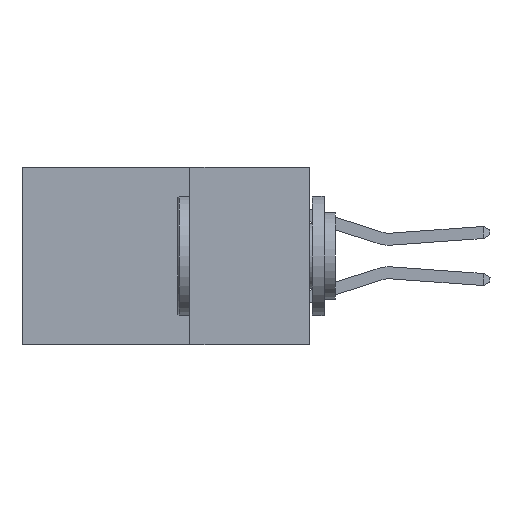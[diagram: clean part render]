
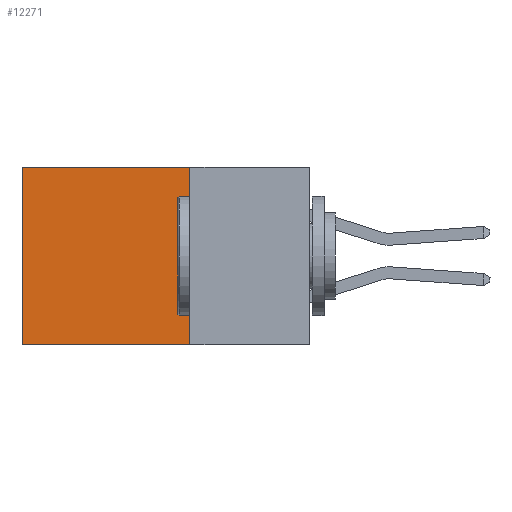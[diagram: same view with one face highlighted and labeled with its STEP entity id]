
A CAD part, left-side view. The second image highlights one B-rep face of the part: STEP entity #12271.
In plain terms, the highlighted planar face has unit normal (-1, 0, 0).
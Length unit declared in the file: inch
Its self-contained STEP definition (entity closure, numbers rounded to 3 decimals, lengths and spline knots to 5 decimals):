
#92 = FACE_OUTER_BOUND ( 'NONE', #14723, .T. ) ;
#436 = CARTESIAN_POINT ( 'NONE',  ( 0.298, 0.25, 0. ) ) ;
#890 = EDGE_CURVE ( 'NONE', #21986, #11920, #2516, .T. ) ;
#1417 = DIRECTION ( 'NONE',  ( 0., 1., 0. ) ) ;
#2134 = DIRECTION ( 'NONE',  ( 0., 0., -1. ) ) ;
#2202 = LINE ( 'NONE', #16030, #6940 ) ;
#2398 = VECTOR ( 'NONE', #1417, 39.37008 ) ;
#2516 = LINE ( 'NONE', #6016, #17220 ) ;
#2739 = CARTESIAN_POINT ( 'NONE',  ( 0.298, 0.25, 0. ) ) ;
#3244 = ORIENTED_EDGE ( 'NONE', *, *, #20453, .T. ) ;
#4372 = ORIENTED_EDGE ( 'NONE', *, *, #22426, .T. ) ;
#6016 = CARTESIAN_POINT ( 'NONE',  ( 0.298, 0.25, 0. ) ) ;
#6204 = VECTOR ( 'NONE', #8843, 39.37008 ) ;
#6940 = VECTOR ( 'NONE', #2134, 39.37008 ) ;
#7319 = LINE ( 'NONE', #21469, #6204 ) ;
#8149 = AXIS2_PLACEMENT_3D ( 'NONE', #436, #19817, #19751 ) ;
#8843 = DIRECTION ( 'NONE',  ( 0., 1., 0. ) ) ;
#8946 = VERTEX_POINT ( 'NONE', #17430 ) ;
#11105 = ORIENTED_EDGE ( 'NONE', *, *, #16914, .F. ) ;
#11837 = VERTEX_POINT ( 'NONE', #18105 ) ;
#11920 = VERTEX_POINT ( 'NONE', #12281 ) ;
#12271 = ADVANCED_FACE ( 'NONE', ( #92 ), #16284, .F. ) ;
#12281 = CARTESIAN_POINT ( 'NONE',  ( 0.298, 0.25, -0.37 ) ) ;
#14723 = EDGE_LOOP ( 'NONE', ( #4372, #11105, #16753, #3244 ) ) ;
#16030 = CARTESIAN_POINT ( 'NONE',  ( 0.298, 0.6, 0. ) ) ;
#16284 = PLANE ( 'NONE',  #8149 ) ;
#16753 = ORIENTED_EDGE ( 'NONE', *, *, #890, .F. ) ;
#16914 = EDGE_CURVE ( 'NONE', #11920, #11837, #21277, .T. ) ;
#17220 = VECTOR ( 'NONE', #18369, 39.37008 ) ;
#17430 = CARTESIAN_POINT ( 'NONE',  ( 0.298, 0.6, 0. ) ) ;
#18105 = CARTESIAN_POINT ( 'NONE',  ( 0.298, 0.6, -0.37 ) ) ;
#18369 = DIRECTION ( 'NONE',  ( 0., 0., -1. ) ) ;
#19751 = DIRECTION ( 'NONE',  ( 0., 0., -1. ) ) ;
#19817 = DIRECTION ( 'NONE',  ( 1., 0., 0. ) ) ;
#20453 = EDGE_CURVE ( 'NONE', #21986, #8946, #7319, .T. ) ;
#20638 = CARTESIAN_POINT ( 'NONE',  ( 0.298, 0.25, -0.37 ) ) ;
#21277 = LINE ( 'NONE', #20638, #2398 ) ;
#21469 = CARTESIAN_POINT ( 'NONE',  ( 0.298, 0.25, 0. ) ) ;
#21986 = VERTEX_POINT ( 'NONE', #2739 ) ;
#22426 = EDGE_CURVE ( 'NONE', #8946, #11837, #2202, .T. ) ;
